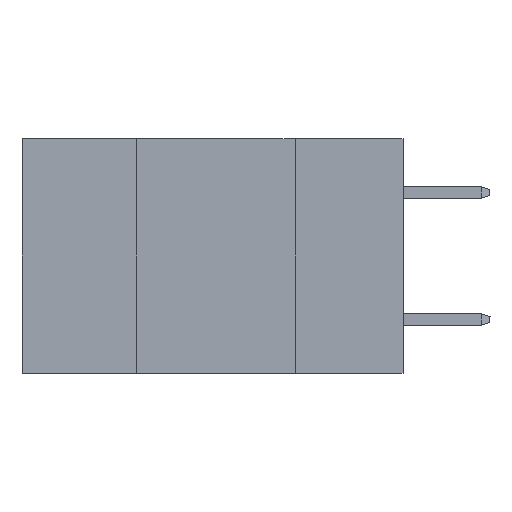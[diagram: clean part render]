
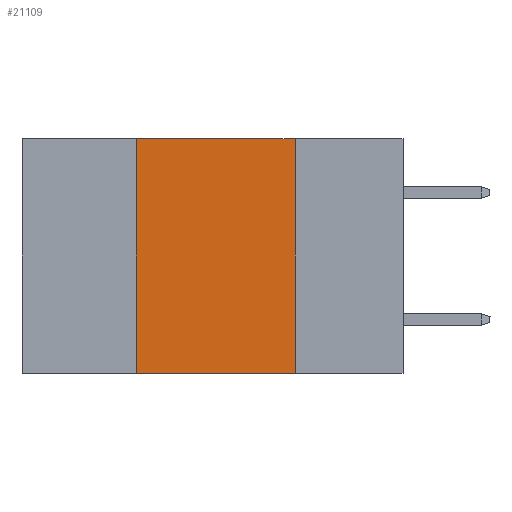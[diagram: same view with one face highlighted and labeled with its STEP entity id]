
A CAD part, left-side view. The second image highlights one B-rep face of the part: STEP entity #21109.
In plain terms, the highlighted planar face has unit normal (-1, 0, 0).
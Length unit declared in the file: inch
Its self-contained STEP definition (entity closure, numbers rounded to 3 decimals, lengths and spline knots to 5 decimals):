
#217 = CARTESIAN_POINT ( 'NONE',  ( 0., 0.17, 0. ) ) ;
#1172 = EDGE_LOOP ( 'NONE', ( #23752, #25023, #12523, #8783 ) ) ;
#1176 = DIRECTION ( 'NONE',  ( 0., -1., 0. ) ) ;
#1651 = FACE_OUTER_BOUND ( 'NONE', #1172, .T. ) ;
#2545 = CARTESIAN_POINT ( 'NONE',  ( 0., 0.42, 0. ) ) ;
#2673 = CARTESIAN_POINT ( 'NONE',  ( 0., 0.42, 0. ) ) ;
#3076 = DIRECTION ( 'NONE',  ( 0., 0., 1. ) ) ;
#3904 = CARTESIAN_POINT ( 'NONE',  ( 0., 0.6, 0. ) ) ;
#5072 = VERTEX_POINT ( 'NONE', #8376 ) ;
#5988 = LINE ( 'NONE', #3904, #11871 ) ;
#6921 = EDGE_CURVE ( 'NONE', #14807, #5072, #26182, .T. ) ;
#6948 = VECTOR ( 'NONE', #14676, 39.37008 ) ;
#8376 = CARTESIAN_POINT ( 'NONE',  ( 0., 0.17, -0.37 ) ) ;
#8783 = ORIENTED_EDGE ( 'NONE', *, *, #6921, .T. ) ;
#11340 = LINE ( 'NONE', #2545, #21025 ) ;
#11609 = CARTESIAN_POINT ( 'NONE',  ( 0., 0.42, -0.37 ) ) ;
#11871 = VECTOR ( 'NONE', #1176, 39.37008 ) ;
#12523 = ORIENTED_EDGE ( 'NONE', *, *, #21573, .F. ) ;
#14167 = CARTESIAN_POINT ( 'NONE',  ( 0., 0.17, 0. ) ) ;
#14676 = DIRECTION ( 'NONE',  ( 0., 0., -1. ) ) ;
#14807 = VERTEX_POINT ( 'NONE', #11609 ) ;
#15448 = DIRECTION ( 'NONE',  ( 0., -1., 0. ) ) ;
#15622 = VERTEX_POINT ( 'NONE', #2673 ) ;
#17445 = VERTEX_POINT ( 'NONE', #14167 ) ;
#20431 = EDGE_CURVE ( 'NONE', #17445, #5072, #22808, .T. ) ;
#20550 = CARTESIAN_POINT ( 'NONE',  ( 0., 0.6, 0. ) ) ;
#20570 = AXIS2_PLACEMENT_3D ( 'NONE', #20550, #26886, #20961 ) ;
#20961 = DIRECTION ( 'NONE',  ( 0., 0., -1. ) ) ;
#21025 = VECTOR ( 'NONE', #3076, 39.37008 ) ;
#21109 = ADVANCED_FACE ( 'NONE', ( #1651 ), #25219, .F. ) ;
#21573 = EDGE_CURVE ( 'NONE', #14807, #15622, #11340, .T. ) ;
#22808 = LINE ( 'NONE', #217, #6948 ) ;
#23752 = ORIENTED_EDGE ( 'NONE', *, *, #20431, .F. ) ;
#23812 = EDGE_CURVE ( 'NONE', #15622, #17445, #5988, .T. ) ;
#24035 = VECTOR ( 'NONE', #15448, 39.37008 ) ;
#25023 = ORIENTED_EDGE ( 'NONE', *, *, #23812, .F. ) ;
#25219 = PLANE ( 'NONE',  #20570 ) ;
#25930 = CARTESIAN_POINT ( 'NONE',  ( 0., 0.6, -0.37 ) ) ;
#26182 = LINE ( 'NONE', #25930, #24035 ) ;
#26886 = DIRECTION ( 'NONE',  ( 1., 0., 0. ) ) ;
